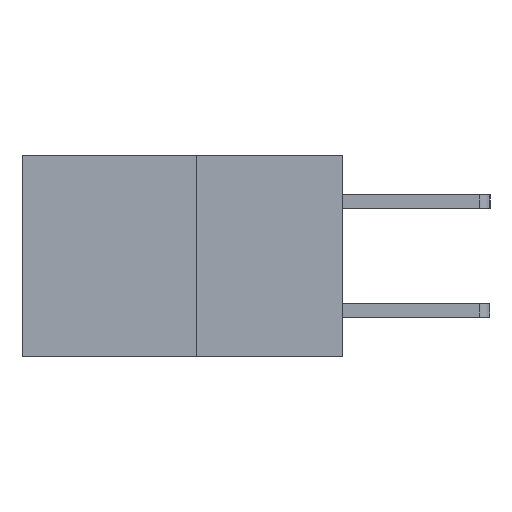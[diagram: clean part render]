
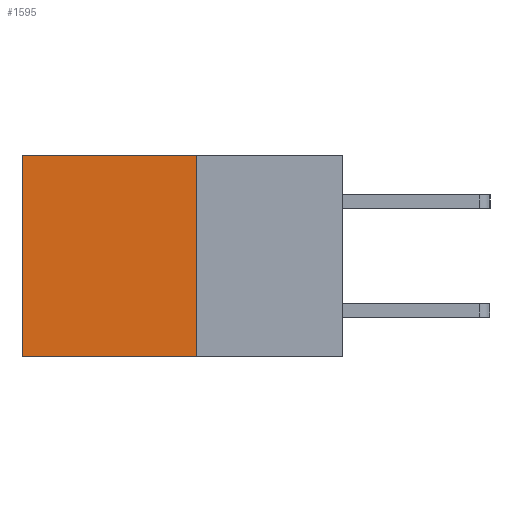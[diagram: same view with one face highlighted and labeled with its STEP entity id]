
A CAD part, left-side view. The second image highlights one B-rep face of the part: STEP entity #1595.
In plain terms, the highlighted planar face has unit normal (-1, 0, 0).
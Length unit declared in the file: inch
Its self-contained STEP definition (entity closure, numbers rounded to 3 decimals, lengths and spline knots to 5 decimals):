
#195 = CARTESIAN_POINT ( 'NONE',  ( 0.277, 0.27, -0.37 ) ) ;
#849 = ORIENTED_EDGE ( 'NONE', *, *, #1261, .T. ) ;
#1261 = EDGE_CURVE ( 'NONE', #5021, #3064, #9039, .T. ) ;
#1466 = EDGE_CURVE ( 'NONE', #7778, #5021, #2784, .T. ) ;
#1595 = ADVANCED_FACE ( 'NONE', ( #9820 ), #2904, .F. ) ;
#1700 = VERTEX_POINT ( 'NONE', #8294 ) ;
#1996 = DIRECTION ( 'NONE',  ( 0., 0., -1. ) ) ;
#2072 = CARTESIAN_POINT ( 'NONE',  ( 0.277, 0.27, -0.37 ) ) ;
#2239 = DIRECTION ( 'NONE',  ( 1., 0., 0. ) ) ;
#2264 = AXIS2_PLACEMENT_3D ( 'NONE', #2691, #2239, #2644 ) ;
#2510 = EDGE_CURVE ( 'NONE', #1700, #3064, #8495, .T. ) ;
#2585 = ORIENTED_EDGE ( 'NONE', *, *, #2510, .F. ) ;
#2644 = DIRECTION ( 'NONE',  ( 0., 0., -1. ) ) ;
#2691 = CARTESIAN_POINT ( 'NONE',  ( 0.277, 0.27, -0.37 ) ) ;
#2784 = LINE ( 'NONE', #5491, #6910 ) ;
#2902 = CARTESIAN_POINT ( 'NONE',  ( 0.277, 0.59, -0.37 ) ) ;
#2904 = PLANE ( 'NONE',  #2264 ) ;
#3064 = VERTEX_POINT ( 'NONE', #2902 ) ;
#3324 = EDGE_LOOP ( 'NONE', ( #849, #2585, #10488, #5388 ) ) ;
#3661 = DIRECTION ( 'NONE',  ( 0., 1., 0. ) ) ;
#4295 = VECTOR ( 'NONE', #3661, 39.37008 ) ;
#4910 = LINE ( 'NONE', #2072, #9119 ) ;
#5021 = VERTEX_POINT ( 'NONE', #9111 ) ;
#5388 = ORIENTED_EDGE ( 'NONE', *, *, #1466, .T. ) ;
#5491 = CARTESIAN_POINT ( 'NONE',  ( 0.277, 0.27, 0. ) ) ;
#6246 = EDGE_CURVE ( 'NONE', #7778, #1700, #4910, .T. ) ;
#6910 = VECTOR ( 'NONE', #9669, 39.37008 ) ;
#7778 = VERTEX_POINT ( 'NONE', #9708 ) ;
#8294 = CARTESIAN_POINT ( 'NONE',  ( 0.277, 0.27, -0.37 ) ) ;
#8495 = LINE ( 'NONE', #195, #4295 ) ;
#8786 = VECTOR ( 'NONE', #9318, 39.37008 ) ;
#9039 = LINE ( 'NONE', #10581, #8786 ) ;
#9111 = CARTESIAN_POINT ( 'NONE',  ( 0.277, 0.59, 0. ) ) ;
#9119 = VECTOR ( 'NONE', #1996, 39.37008 ) ;
#9318 = DIRECTION ( 'NONE',  ( 0., 0., -1. ) ) ;
#9669 = DIRECTION ( 'NONE',  ( 0., 1., 0. ) ) ;
#9708 = CARTESIAN_POINT ( 'NONE',  ( 0.277, 0.27, 0. ) ) ;
#9820 = FACE_OUTER_BOUND ( 'NONE', #3324, .T. ) ;
#10488 = ORIENTED_EDGE ( 'NONE', *, *, #6246, .F. ) ;
#10581 = CARTESIAN_POINT ( 'NONE',  ( 0.277, 0.59, -0.37 ) ) ;
